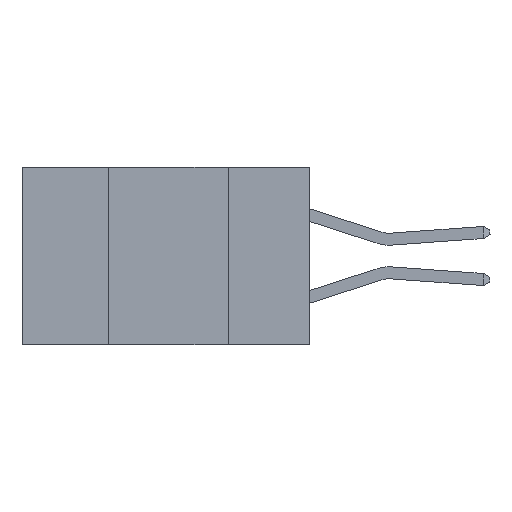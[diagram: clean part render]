
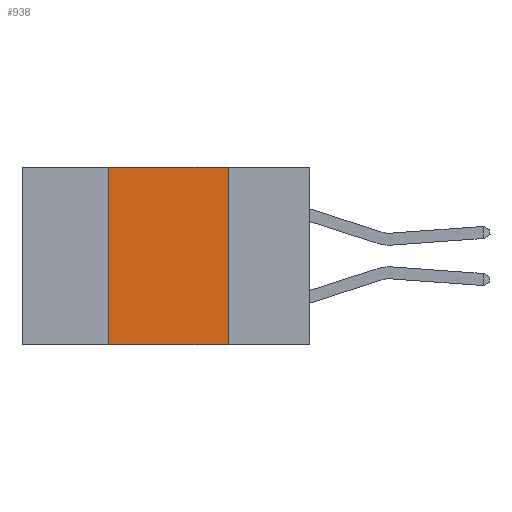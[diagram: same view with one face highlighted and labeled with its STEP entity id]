
A CAD part, left-side view. The second image highlights one B-rep face of the part: STEP entity #938.
In plain terms, the highlighted planar face has unit normal (-1, 0, 0).
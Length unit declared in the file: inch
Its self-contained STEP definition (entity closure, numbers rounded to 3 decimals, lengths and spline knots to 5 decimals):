
#636 = CARTESIAN_POINT ( 'NONE',  ( 0., 0.17, -0.37 ) ) ;
#694 = CARTESIAN_POINT ( 'NONE',  ( 0., 0.42, 0. ) ) ;
#849 = EDGE_CURVE ( 'NONE', #4145, #7556, #4758, .T. ) ;
#938 = ADVANCED_FACE ( 'NONE', ( #3857 ), #4634, .F. ) ;
#1011 = CARTESIAN_POINT ( 'NONE',  ( 0., 0.42, -0.37 ) ) ;
#1345 = ORIENTED_EDGE ( 'NONE', *, *, #849, .F. ) ;
#1407 = EDGE_CURVE ( 'NONE', #5904, #2937, #1749, .T. ) ;
#1460 = CARTESIAN_POINT ( 'NONE',  ( 0., 0.6, 0. ) ) ;
#1612 = ORIENTED_EDGE ( 'NONE', *, *, #9067, .T. ) ;
#1749 = LINE ( 'NONE', #636, #8912 ) ;
#1901 = DIRECTION ( 'NONE',  ( 0., -1., 0. ) ) ;
#2227 = DIRECTION ( 'NONE',  ( 0., 0., -1. ) ) ;
#2491 = EDGE_CURVE ( 'NONE', #7556, #5904, #3816, .T. ) ;
#2937 = VERTEX_POINT ( 'NONE', #5120 ) ;
#3065 = CARTESIAN_POINT ( 'NONE',  ( 0., 0.42, -0.37 ) ) ;
#3816 = LINE ( 'NONE', #1460, #8972 ) ;
#3857 = FACE_OUTER_BOUND ( 'NONE', #5996, .T. ) ;
#3910 = DIRECTION ( 'NONE',  ( 1., 0., 0. ) ) ;
#4145 = VERTEX_POINT ( 'NONE', #3065 ) ;
#4634 = PLANE ( 'NONE',  #7672 ) ;
#4758 = LINE ( 'NONE', #1011, #6809 ) ;
#5120 = CARTESIAN_POINT ( 'NONE',  ( 0., 0.17, -0.37 ) ) ;
#5558 = CARTESIAN_POINT ( 'NONE',  ( 0., 0.6, 0. ) ) ;
#5904 = VERTEX_POINT ( 'NONE', #6617 ) ;
#5996 = EDGE_LOOP ( 'NONE', ( #6879, #8600, #1345, #1612 ) ) ;
#6155 = DIRECTION ( 'NONE',  ( 0., -1., 0. ) ) ;
#6334 = DIRECTION ( 'NONE',  ( 0., 0., 1. ) ) ;
#6617 = CARTESIAN_POINT ( 'NONE',  ( 0., 0.17, 0. ) ) ;
#6809 = VECTOR ( 'NONE', #6334, 39.37008 ) ;
#6879 = ORIENTED_EDGE ( 'NONE', *, *, #1407, .F. ) ;
#7055 = LINE ( 'NONE', #8757, #8780 ) ;
#7556 = VERTEX_POINT ( 'NONE', #694 ) ;
#7672 = AXIS2_PLACEMENT_3D ( 'NONE', #5558, #3910, #2227 ) ;
#8173 = DIRECTION ( 'NONE',  ( 0., 0., -1. ) ) ;
#8600 = ORIENTED_EDGE ( 'NONE', *, *, #2491, .F. ) ;
#8757 = CARTESIAN_POINT ( 'NONE',  ( 0., 0.6, -0.37 ) ) ;
#8780 = VECTOR ( 'NONE', #6155, 39.37008 ) ;
#8912 = VECTOR ( 'NONE', #8173, 39.37008 ) ;
#8972 = VECTOR ( 'NONE', #1901, 39.37008 ) ;
#9067 = EDGE_CURVE ( 'NONE', #4145, #2937, #7055, .T. ) ;
